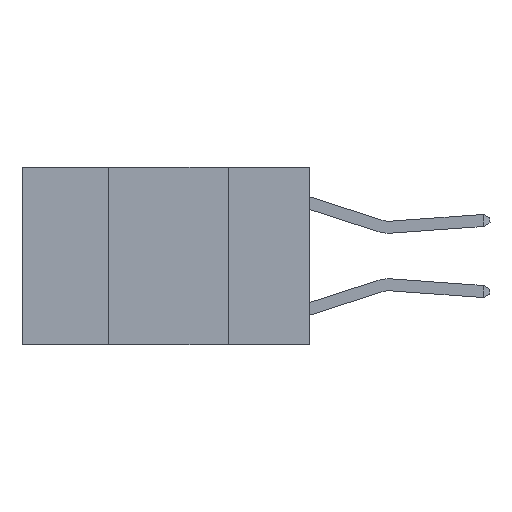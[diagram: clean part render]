
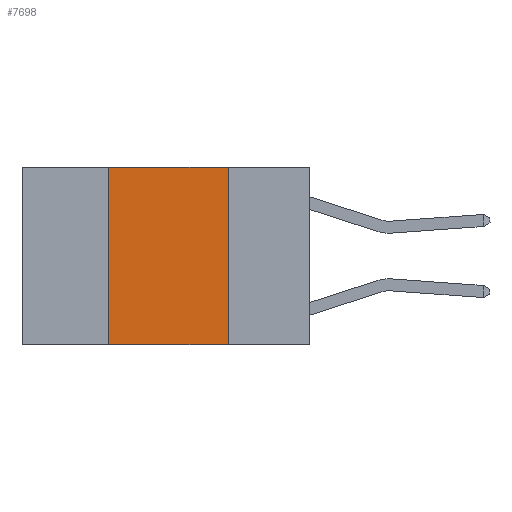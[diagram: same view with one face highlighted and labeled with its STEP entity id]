
A CAD part, left-side view. The second image highlights one B-rep face of the part: STEP entity #7698.
In plain terms, the highlighted planar face has unit normal (-1, 0, 0).
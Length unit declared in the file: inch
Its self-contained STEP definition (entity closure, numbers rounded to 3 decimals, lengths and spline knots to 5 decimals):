
#321 = VECTOR ( 'NONE', #23147, 39.37008 ) ;
#3369 = DIRECTION ( 'NONE',  ( 0., 0., -1. ) ) ;
#4075 = ORIENTED_EDGE ( 'NONE', *, *, #9851, .F. ) ;
#4140 = VECTOR ( 'NONE', #4215, 39.37008 ) ;
#4215 = DIRECTION ( 'NONE',  ( 0., 0., 1. ) ) ;
#4782 = EDGE_LOOP ( 'NONE', ( #24382, #4075, #25568, #10568 ) ) ;
#4826 = EDGE_CURVE ( 'NONE', #16363, #18555, #11599, .T. ) ;
#5335 = CARTESIAN_POINT ( 'NONE',  ( 0., 0.6, 0. ) ) ;
#6014 = CARTESIAN_POINT ( 'NONE',  ( 0., 0.42, 0. ) ) ;
#7698 = ADVANCED_FACE ( 'NONE', ( #24906 ), #23021, .F. ) ;
#8174 = CARTESIAN_POINT ( 'NONE',  ( 0., 0.42, 0. ) ) ;
#8785 = LINE ( 'NONE', #8174, #4140 ) ;
#9264 = CARTESIAN_POINT ( 'NONE',  ( 0., 0.6, 0. ) ) ;
#9529 = VECTOR ( 'NONE', #25549, 39.37008 ) ;
#9713 = LINE ( 'NONE', #5335, #19623 ) ;
#9851 = EDGE_CURVE ( 'NONE', #12899, #24171, #9713, .T. ) ;
#10135 = EDGE_CURVE ( 'NONE', #16363, #12899, #8785, .T. ) ;
#10568 = ORIENTED_EDGE ( 'NONE', *, *, #4826, .T. ) ;
#11599 = LINE ( 'NONE', #25068, #321 ) ;
#12608 = CARTESIAN_POINT ( 'NONE',  ( 0., 0.42, -0.37 ) ) ;
#12899 = VERTEX_POINT ( 'NONE', #6014 ) ;
#14142 = EDGE_CURVE ( 'NONE', #24171, #18555, #14817, .T. ) ;
#14817 = LINE ( 'NONE', #19663, #9529 ) ;
#15247 = DIRECTION ( 'NONE',  ( 1., 0., 0. ) ) ;
#16363 = VERTEX_POINT ( 'NONE', #12608 ) ;
#16928 = CARTESIAN_POINT ( 'NONE',  ( 0., 0.17, 0. ) ) ;
#18233 = AXIS2_PLACEMENT_3D ( 'NONE', #9264, #15247, #3369 ) ;
#18555 = VERTEX_POINT ( 'NONE', #24870 ) ;
#19623 = VECTOR ( 'NONE', #23088, 39.37008 ) ;
#19663 = CARTESIAN_POINT ( 'NONE',  ( 0., 0.17, 0. ) ) ;
#23021 = PLANE ( 'NONE',  #18233 ) ;
#23088 = DIRECTION ( 'NONE',  ( 0., -1., 0. ) ) ;
#23147 = DIRECTION ( 'NONE',  ( 0., -1., 0. ) ) ;
#24171 = VERTEX_POINT ( 'NONE', #16928 ) ;
#24382 = ORIENTED_EDGE ( 'NONE', *, *, #14142, .F. ) ;
#24870 = CARTESIAN_POINT ( 'NONE',  ( 0., 0.17, -0.37 ) ) ;
#24906 = FACE_OUTER_BOUND ( 'NONE', #4782, .T. ) ;
#25068 = CARTESIAN_POINT ( 'NONE',  ( 0., 0.6, -0.37 ) ) ;
#25549 = DIRECTION ( 'NONE',  ( 0., 0., -1. ) ) ;
#25568 = ORIENTED_EDGE ( 'NONE', *, *, #10135, .F. ) ;
